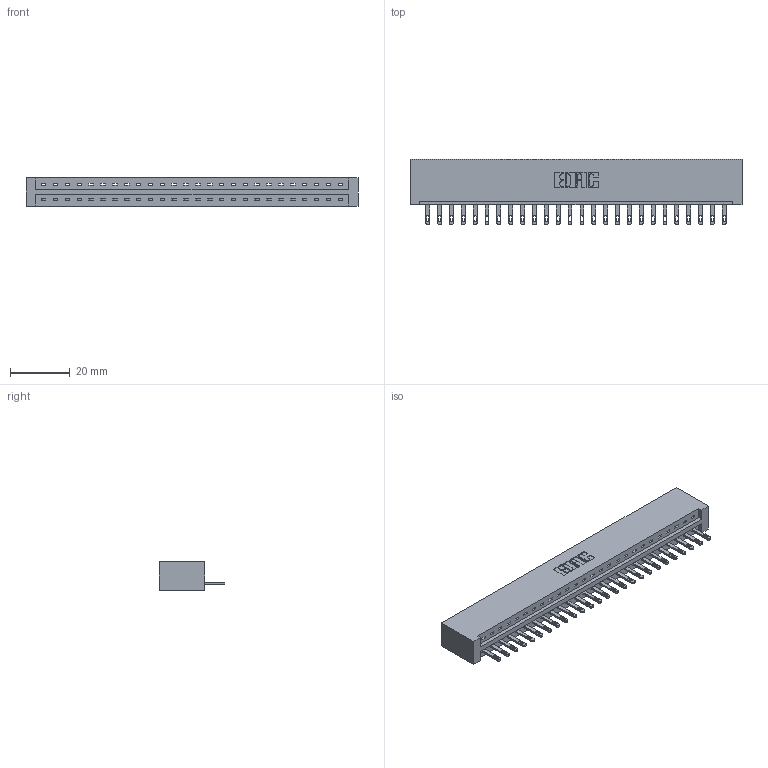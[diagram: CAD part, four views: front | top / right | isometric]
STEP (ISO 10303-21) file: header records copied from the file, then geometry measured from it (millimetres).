
FILE_DESCRIPTION (( 'STEP AP203' ), '1' );
FILE_NAME ('337-026-500-101.STEP', '2018-08-06T03:41:57', ( '' ), ( '' ), 'SwSTEP 2.0', 'SolidWorks 2016', '' );
FILE_SCHEMA (( 'CONFIG_CONTROL_DESIGN' ));
Length unit declared in the file: inch
Products named in the file (3): 337 Part_No Mounting Lugs; 345-292-001_345-293-100; 337-026-500-101
Assembly tree (27 placements, depth 2):
  337-026-500-101
    337 Part_No Mounting Lugs
    345-292-001_345-293-100  x26
Bounding box: 110.9 x 21.85 x 9.4 mm (x, y, z)
Volume: 12080.4 mm3; surface area: 12436.7 mm2
Topology: 27 solids, 27 shells, 1614 faces, 4967 edges, 3310 vertices
Faces by surface type: plane 1106, cylinder 508
Entity records: 21049 total; most frequent: CARTESIAN_POINT 3672, ORIENTED_EDGE 3634, DIRECTION 3117, EDGE_CURVE 1817, LINE 1693, VECTOR 1693, VERTEX_POINT 1210, AXIS2_PLACEMENT_3D 712
